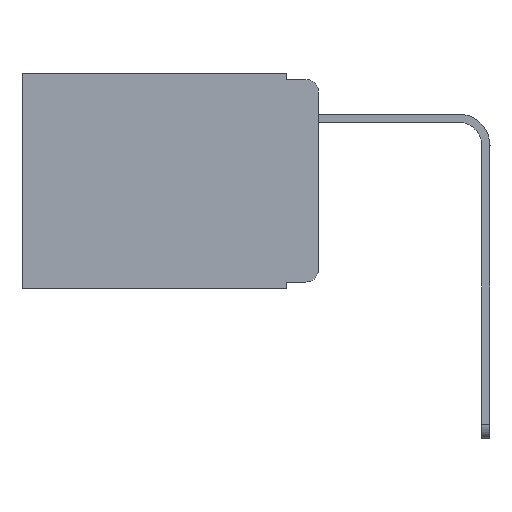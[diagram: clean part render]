
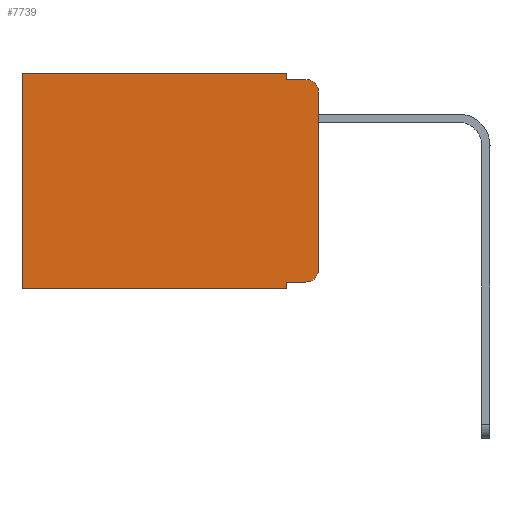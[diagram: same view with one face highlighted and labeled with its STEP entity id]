
A CAD part, left-side view. The second image highlights one B-rep face of the part: STEP entity #7739.
In plain terms, the highlighted planar face has unit normal (-1, 0, 0).
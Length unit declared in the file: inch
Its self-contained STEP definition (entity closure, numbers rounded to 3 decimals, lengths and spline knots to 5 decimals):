
#230 = EDGE_CURVE ( 'NONE', #17525, #13806, #4318, .T. ) ;
#481 = DIRECTION ( 'NONE',  ( 0., -1., 0. ) ) ;
#501 = CARTESIAN_POINT ( 'NONE',  ( 0.298, 0.051, 0. ) ) ;
#583 = CARTESIAN_POINT ( 'NONE',  ( 0.298, 0.473, -0.343 ) ) ;
#1313 = CARTESIAN_POINT ( 'NONE',  ( 0.298, 0.051, -0.333 ) ) ;
#1552 = DIRECTION ( 'NONE',  ( 0., 1., 0. ) ) ;
#1559 = EDGE_CURVE ( 'NONE', #6392, #18357, #18458, .T. ) ;
#1664 = ORIENTED_EDGE ( 'NONE', *, *, #17699, .T. ) ;
#1676 = FACE_OUTER_BOUND ( 'NONE', #22065, .T. ) ;
#1932 = CIRCLE ( 'NONE', #9791, 0.02 ) ;
#2156 = ORIENTED_EDGE ( 'NONE', *, *, #5132, .F. ) ;
#2534 = CARTESIAN_POINT ( 'NONE',  ( 0.298, 0.473, 0. ) ) ;
#2579 = CARTESIAN_POINT ( 'NONE',  ( 0.298, 0., 0. ) ) ;
#2580 = ORIENTED_EDGE ( 'NONE', *, *, #7925, .T. ) ;
#2797 = CARTESIAN_POINT ( 'NONE',  ( 0.298, 0., -0.313 ) ) ;
#3130 = VERTEX_POINT ( 'NONE', #2534 ) ;
#4072 = DIRECTION ( 'NONE',  ( 1., 0., 0. ) ) ;
#4318 = LINE ( 'NONE', #2579, #17697 ) ;
#4683 = VECTOR ( 'NONE', #19702, 39.37008 ) ;
#5132 = EDGE_CURVE ( 'NONE', #7768, #19187, #22197, .T. ) ;
#5945 = DIRECTION ( 'NONE',  ( 0., 0., -1. ) ) ;
#6181 = LINE ( 'NONE', #9888, #11379 ) ;
#6363 = LINE ( 'NONE', #7634, #4683 ) ;
#6376 = DIRECTION ( 'NONE',  ( 0., 1., 0. ) ) ;
#6392 = VERTEX_POINT ( 'NONE', #17313 ) ;
#6499 = CARTESIAN_POINT ( 'NONE',  ( 0.298, 0.051, -0.01 ) ) ;
#7265 = CARTESIAN_POINT ( 'NONE',  ( 0.298, 0., -0.03 ) ) ;
#7284 = DIRECTION ( 'NONE',  ( -1., 0., 0. ) ) ;
#7508 = ORIENTED_EDGE ( 'NONE', *, *, #17757, .T. ) ;
#7634 = CARTESIAN_POINT ( 'NONE',  ( 0.298, 0.473, 0. ) ) ;
#7739 = ADVANCED_FACE ( 'NONE', ( #1676 ), #19746, .F. ) ;
#7768 = VERTEX_POINT ( 'NONE', #501 ) ;
#7925 = EDGE_CURVE ( 'NONE', #22023, #13806, #1932, .T. ) ;
#7993 = EDGE_CURVE ( 'NONE', #19187, #13912, #9034, .T. ) ;
#8146 = CARTESIAN_POINT ( 'NONE',  ( 0.298, 0.051, -0.333 ) ) ;
#9034 = LINE ( 'NONE', #12766, #17493 ) ;
#9454 = DIRECTION ( 'NONE',  ( -1., 0., 0. ) ) ;
#9637 = CARTESIAN_POINT ( 'NONE',  ( 0.298, 0.051, 0. ) ) ;
#9791 = AXIS2_PLACEMENT_3D ( 'NONE', #17794, #7284, #17492 ) ;
#9888 = CARTESIAN_POINT ( 'NONE',  ( 0.298, 0., 0. ) ) ;
#9994 = VECTOR ( 'NONE', #1552, 39.37008 ) ;
#10364 = ORIENTED_EDGE ( 'NONE', *, *, #12505, .T. ) ;
#10406 = VERTEX_POINT ( 'NONE', #8146 ) ;
#10666 = AXIS2_PLACEMENT_3D ( 'NONE', #14375, #4072, #21417 ) ;
#10777 = ORIENTED_EDGE ( 'NONE', *, *, #1559, .F. ) ;
#11300 = EDGE_CURVE ( 'NONE', #10406, #6392, #17540, .T. ) ;
#11379 = VECTOR ( 'NONE', #6376, 39.37008 ) ;
#11959 = ORIENTED_EDGE ( 'NONE', *, *, #7993, .F. ) ;
#12330 = CARTESIAN_POINT ( 'NONE',  ( 0.298, 0., -0.343 ) ) ;
#12374 = VECTOR ( 'NONE', #19820, 39.37008 ) ;
#12505 = EDGE_CURVE ( 'NONE', #10406, #22023, #22530, .T. ) ;
#12766 = CARTESIAN_POINT ( 'NONE',  ( 0.298, 0.051, -0.01 ) ) ;
#12784 = CARTESIAN_POINT ( 'NONE',  ( 0.298, 0.051, 0. ) ) ;
#13806 = VERTEX_POINT ( 'NONE', #2797 ) ;
#13912 = VERTEX_POINT ( 'NONE', #18522 ) ;
#14163 = ORIENTED_EDGE ( 'NONE', *, *, #16733, .T. ) ;
#14375 = CARTESIAN_POINT ( 'NONE',  ( 0.298, 0., 0. ) ) ;
#14859 = DIRECTION ( 'NONE',  ( 0., 0., -1. ) ) ;
#14963 = VECTOR ( 'NONE', #16567, 39.37008 ) ;
#15623 = CARTESIAN_POINT ( 'NONE',  ( 0.298, 0.02, -0.333 ) ) ;
#16194 = AXIS2_PLACEMENT_3D ( 'NONE', #18299, #9454, #5945 ) ;
#16567 = DIRECTION ( 'NONE',  ( 0., 0., -1. ) ) ;
#16733 = EDGE_CURVE ( 'NONE', #7768, #3130, #6181, .T. ) ;
#16876 = DIRECTION ( 'NONE',  ( 0., -1., 0. ) ) ;
#17313 = CARTESIAN_POINT ( 'NONE',  ( 0.298, 0.051, -0.343 ) ) ;
#17492 = DIRECTION ( 'NONE',  ( 0., 0., -1. ) ) ;
#17493 = VECTOR ( 'NONE', #481, 39.37008 ) ;
#17525 = VERTEX_POINT ( 'NONE', #7265 ) ;
#17540 = LINE ( 'NONE', #12784, #12374 ) ;
#17697 = VECTOR ( 'NONE', #14859, 39.37008 ) ;
#17699 = EDGE_CURVE ( 'NONE', #3130, #18357, #6363, .T. ) ;
#17757 = EDGE_CURVE ( 'NONE', #17525, #13912, #22095, .T. ) ;
#17794 = CARTESIAN_POINT ( 'NONE',  ( 0.298, 0.02, -0.313 ) ) ;
#18130 = ORIENTED_EDGE ( 'NONE', *, *, #11300, .F. ) ;
#18299 = CARTESIAN_POINT ( 'NONE',  ( 0.298, 0.02, -0.03 ) ) ;
#18357 = VERTEX_POINT ( 'NONE', #583 ) ;
#18458 = LINE ( 'NONE', #12330, #9994 ) ;
#18522 = CARTESIAN_POINT ( 'NONE',  ( 0.298, 0.02, -0.01 ) ) ;
#19187 = VERTEX_POINT ( 'NONE', #6499 ) ;
#19702 = DIRECTION ( 'NONE',  ( 0., 0., -1. ) ) ;
#19710 = ORIENTED_EDGE ( 'NONE', *, *, #230, .F. ) ;
#19746 = PLANE ( 'NONE',  #10666 ) ;
#19782 = VECTOR ( 'NONE', #16876, 39.37008 ) ;
#19820 = DIRECTION ( 'NONE',  ( 0., 0., -1. ) ) ;
#21417 = DIRECTION ( 'NONE',  ( 0., 0., -1. ) ) ;
#22023 = VERTEX_POINT ( 'NONE', #15623 ) ;
#22065 = EDGE_LOOP ( 'NONE', ( #19710, #7508, #11959, #2156, #14163, #1664, #10777, #18130, #10364, #2580 ) ) ;
#22095 = CIRCLE ( 'NONE', #16194, 0.02 ) ;
#22197 = LINE ( 'NONE', #9637, #14963 ) ;
#22530 = LINE ( 'NONE', #1313, #19782 ) ;
